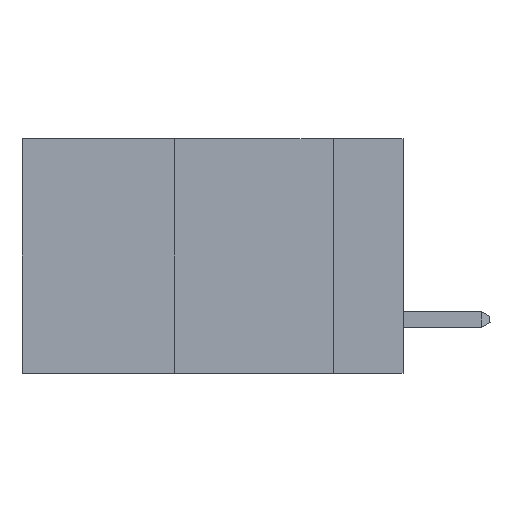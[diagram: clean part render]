
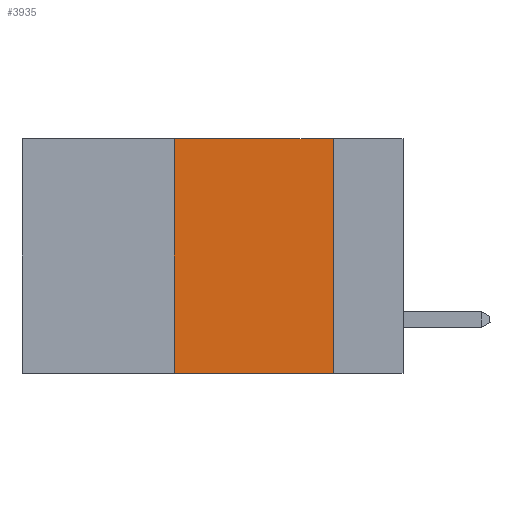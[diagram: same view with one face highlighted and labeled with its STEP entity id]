
A CAD part, left-side view. The second image highlights one B-rep face of the part: STEP entity #3935.
In plain terms, the highlighted planar face has unit normal (-1, 0, 0).
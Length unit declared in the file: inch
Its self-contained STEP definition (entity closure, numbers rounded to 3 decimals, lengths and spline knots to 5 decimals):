
#187 = VECTOR ( 'NONE', #3467, 39.37008 ) ;
#510 = ORIENTED_EDGE ( 'NONE', *, *, #10846, .F. ) ;
#1381 = CARTESIAN_POINT ( 'NONE',  ( 0., 0.36, -0.37 ) ) ;
#1900 = EDGE_CURVE ( 'NONE', #4468, #10696, #10819, .T. ) ;
#2241 = LINE ( 'NONE', #5935, #187 ) ;
#3069 = EDGE_CURVE ( 'NONE', #6628, #4207, #6172, .T. ) ;
#3252 = CARTESIAN_POINT ( 'NONE',  ( 0., 0.11, 0. ) ) ;
#3288 = CARTESIAN_POINT ( 'NONE',  ( 0., 0.6, 0. ) ) ;
#3467 = DIRECTION ( 'NONE',  ( 0., -1., 0. ) ) ;
#3934 = ORIENTED_EDGE ( 'NONE', *, *, #4003, .T. ) ;
#3935 = ADVANCED_FACE ( 'NONE', ( #9149 ), #10237, .F. ) ;
#4003 = EDGE_CURVE ( 'NONE', #4468, #4207, #2241, .T. ) ;
#4207 = VERTEX_POINT ( 'NONE', #8006 ) ;
#4468 = VERTEX_POINT ( 'NONE', #1381 ) ;
#5183 = VECTOR ( 'NONE', #10883, 39.37008 ) ;
#5935 = CARTESIAN_POINT ( 'NONE',  ( 0., 0.6, -0.37 ) ) ;
#6172 = LINE ( 'NONE', #10349, #9323 ) ;
#6330 = VECTOR ( 'NONE', #7169, 39.37008 ) ;
#6528 = EDGE_LOOP ( 'NONE', ( #7021, #510, #11292, #3934 ) ) ;
#6628 = VERTEX_POINT ( 'NONE', #3252 ) ;
#7021 = ORIENTED_EDGE ( 'NONE', *, *, #3069, .F. ) ;
#7072 = LINE ( 'NONE', #3288, #6330 ) ;
#7169 = DIRECTION ( 'NONE',  ( 0., -1., 0. ) ) ;
#7994 = AXIS2_PLACEMENT_3D ( 'NONE', #8272, #11124, #11160 ) ;
#8006 = CARTESIAN_POINT ( 'NONE',  ( 0., 0.11, -0.37 ) ) ;
#8272 = CARTESIAN_POINT ( 'NONE',  ( 0., 0.6, 0. ) ) ;
#8754 = DIRECTION ( 'NONE',  ( 0., 0., -1. ) ) ;
#8829 = CARTESIAN_POINT ( 'NONE',  ( 0., 0.36, 0. ) ) ;
#9051 = CARTESIAN_POINT ( 'NONE',  ( 0., 0.36, 0. ) ) ;
#9149 = FACE_OUTER_BOUND ( 'NONE', #6528, .T. ) ;
#9323 = VECTOR ( 'NONE', #8754, 39.37008 ) ;
#10237 = PLANE ( 'NONE',  #7994 ) ;
#10349 = CARTESIAN_POINT ( 'NONE',  ( 0., 0.11, 0. ) ) ;
#10696 = VERTEX_POINT ( 'NONE', #8829 ) ;
#10819 = LINE ( 'NONE', #9051, #5183 ) ;
#10846 = EDGE_CURVE ( 'NONE', #10696, #6628, #7072, .T. ) ;
#10883 = DIRECTION ( 'NONE',  ( 0., 0., 1. ) ) ;
#11124 = DIRECTION ( 'NONE',  ( 1., 0., 0. ) ) ;
#11160 = DIRECTION ( 'NONE',  ( 0., 0., -1. ) ) ;
#11292 = ORIENTED_EDGE ( 'NONE', *, *, #1900, .F. ) ;
